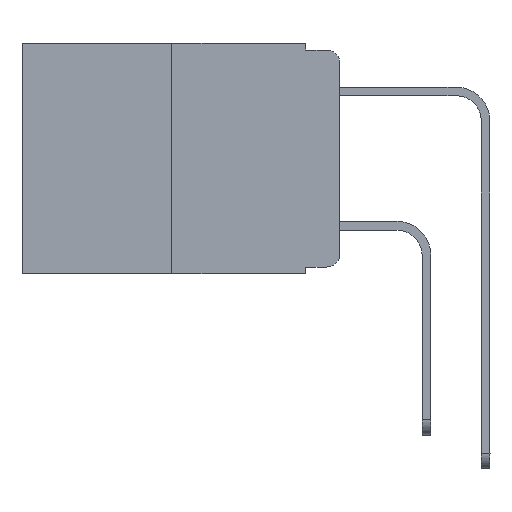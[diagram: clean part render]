
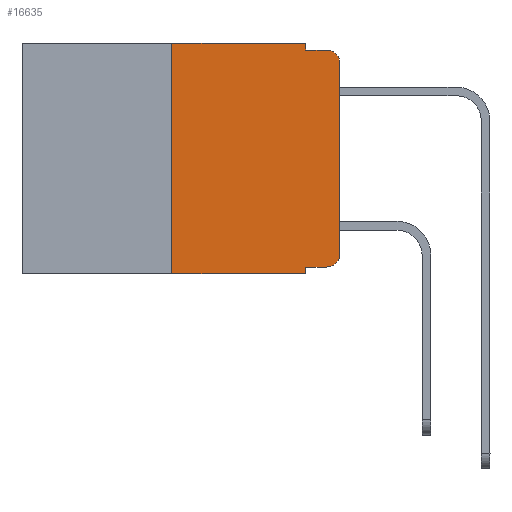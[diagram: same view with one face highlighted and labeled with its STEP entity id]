
A CAD part, left-side view. The second image highlights one B-rep face of the part: STEP entity #16635.
In plain terms, the highlighted planar face has unit normal (-1, 0, 0).
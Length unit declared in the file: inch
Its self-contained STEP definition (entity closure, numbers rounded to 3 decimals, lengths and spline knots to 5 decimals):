
#30 = ORIENTED_EDGE ( 'NONE', *, *, #8420, .T. ) ;
#124 = EDGE_CURVE ( 'NONE', #16669, #15917, #20163, .T. ) ;
#125 = DIRECTION ( 'NONE',  ( 0., 0., 1. ) ) ;
#176 = CARTESIAN_POINT ( 'NONE',  ( 0., 0.051, -0.01 ) ) ;
#660 = ORIENTED_EDGE ( 'NONE', *, *, #124, .T. ) ;
#1376 = CARTESIAN_POINT ( 'NONE',  ( 0., 0.25, 0. ) ) ;
#1667 = CARTESIAN_POINT ( 'NONE',  ( 0., 0.02, -0.313 ) ) ;
#3155 = CARTESIAN_POINT ( 'NONE',  ( 0., 0.051, 0. ) ) ;
#3241 = CARTESIAN_POINT ( 'NONE',  ( 0., 0.051, -0.343 ) ) ;
#3361 = LINE ( 'NONE', #5131, #3373 ) ;
#3373 = VECTOR ( 'NONE', #14288, 39.37008 ) ;
#3450 = DIRECTION ( 'NONE',  ( 1., 0., 0. ) ) ;
#3804 = VERTEX_POINT ( 'NONE', #176 ) ;
#4128 = DIRECTION ( 'NONE',  ( 0., -1., 0. ) ) ;
#4279 = EDGE_CURVE ( 'NONE', #8288, #5903, #12335, .T. ) ;
#4603 = VERTEX_POINT ( 'NONE', #13559 ) ;
#4614 = DIRECTION ( 'NONE',  ( 0., 0., -1. ) ) ;
#4744 = DIRECTION ( 'NONE',  ( 0., 0., -1. ) ) ;
#4758 = DIRECTION ( 'NONE',  ( 0., 0., 1. ) ) ;
#4771 = CARTESIAN_POINT ( 'NONE',  ( 0., 0.051, -0.333 ) ) ;
#5011 = PLANE ( 'NONE',  #13965 ) ;
#5131 = CARTESIAN_POINT ( 'NONE',  ( 0., 0.051, -0.01 ) ) ;
#5778 = AXIS2_PLACEMENT_3D ( 'NONE', #6007, #12176, #4744 ) ;
#5903 = VERTEX_POINT ( 'NONE', #3241 ) ;
#5946 = EDGE_CURVE ( 'NONE', #18652, #8633, #12513, .T. ) ;
#6007 = CARTESIAN_POINT ( 'NONE',  ( 0., 0.02, -0.03 ) ) ;
#6169 = EDGE_CURVE ( 'NONE', #15917, #17585, #12990, .T. ) ;
#6672 = EDGE_LOOP ( 'NONE', ( #660, #14178, #7880, #9277, #15893, #14570, #6991, #7124, #15206, #30 ) ) ;
#6991 = ORIENTED_EDGE ( 'NONE', *, *, #9196, .T. ) ;
#7124 = ORIENTED_EDGE ( 'NONE', *, *, #4279, .F. ) ;
#7330 = LINE ( 'NONE', #19630, #10176 ) ;
#7664 = CARTESIAN_POINT ( 'NONE',  ( 0., 0.25, -0.343 ) ) ;
#7880 = ORIENTED_EDGE ( 'NONE', *, *, #9917, .F. ) ;
#7937 = CARTESIAN_POINT ( 'NONE',  ( 0., 0.02, -0.01 ) ) ;
#8288 = VERTEX_POINT ( 'NONE', #16791 ) ;
#8420 = EDGE_CURVE ( 'NONE', #15781, #16669, #13388, .T. ) ;
#8600 = CARTESIAN_POINT ( 'NONE',  ( 0., 0., -0.313 ) ) ;
#8633 = VERTEX_POINT ( 'NONE', #11383 ) ;
#9075 = CARTESIAN_POINT ( 'NONE',  ( 0., 0.473, -0.343 ) ) ;
#9170 = EDGE_CURVE ( 'NONE', #8633, #4603, #7330, .T. ) ;
#9196 = EDGE_CURVE ( 'NONE', #18652, #5903, #16712, .T. ) ;
#9277 = ORIENTED_EDGE ( 'NONE', *, *, #15450, .F. ) ;
#9739 = DIRECTION ( 'NONE',  ( 0., 0., -1. ) ) ;
#9917 = EDGE_CURVE ( 'NONE', #3804, #17585, #3361, .T. ) ;
#10026 = VECTOR ( 'NONE', #11053, 39.37008 ) ;
#10176 = VECTOR ( 'NONE', #20034, 39.37008 ) ;
#10424 = AXIS2_PLACEMENT_3D ( 'NONE', #1667, #20210, #16883 ) ;
#11053 = DIRECTION ( 'NONE',  ( 0., -1., 0. ) ) ;
#11383 = CARTESIAN_POINT ( 'NONE',  ( 0., 0.25, 0. ) ) ;
#12176 = DIRECTION ( 'NONE',  ( -1., 0., 0. ) ) ;
#12335 = LINE ( 'NONE', #3155, #20222 ) ;
#12513 = LINE ( 'NONE', #1376, #14949 ) ;
#12990 = CIRCLE ( 'NONE', #5778, 0.02 ) ;
#13325 = CARTESIAN_POINT ( 'NONE',  ( 0., 0.051, 0. ) ) ;
#13388 = CIRCLE ( 'NONE', #10424, 0.02 ) ;
#13559 = CARTESIAN_POINT ( 'NONE',  ( 0., 0.051, 0. ) ) ;
#13585 = VECTOR ( 'NONE', #14992, 39.37008 ) ;
#13965 = AXIS2_PLACEMENT_3D ( 'NONE', #17584, #3450, #9739 ) ;
#14035 = CARTESIAN_POINT ( 'NONE',  ( 0., 0., 0. ) ) ;
#14117 = VECTOR ( 'NONE', #4128, 39.37008 ) ;
#14178 = ORIENTED_EDGE ( 'NONE', *, *, #6169, .T. ) ;
#14288 = DIRECTION ( 'NONE',  ( 0., -1., 0. ) ) ;
#14570 = ORIENTED_EDGE ( 'NONE', *, *, #5946, .F. ) ;
#14949 = VECTOR ( 'NONE', #125, 39.37008 ) ;
#14992 = DIRECTION ( 'NONE',  ( 0., 0., -1. ) ) ;
#15206 = ORIENTED_EDGE ( 'NONE', *, *, #17102, .T. ) ;
#15270 = CARTESIAN_POINT ( 'NONE',  ( 0., 0., -0.03 ) ) ;
#15450 = EDGE_CURVE ( 'NONE', #4603, #3804, #19770, .T. ) ;
#15781 = VERTEX_POINT ( 'NONE', #16013 ) ;
#15893 = ORIENTED_EDGE ( 'NONE', *, *, #9170, .F. ) ;
#15917 = VERTEX_POINT ( 'NONE', #15270 ) ;
#16013 = CARTESIAN_POINT ( 'NONE',  ( 0., 0.02, -0.333 ) ) ;
#16635 = ADVANCED_FACE ( 'NONE', ( #19147 ), #5011, .F. ) ;
#16669 = VERTEX_POINT ( 'NONE', #8600 ) ;
#16712 = LINE ( 'NONE', #9075, #14117 ) ;
#16791 = CARTESIAN_POINT ( 'NONE',  ( 0., 0.051, -0.333 ) ) ;
#16883 = DIRECTION ( 'NONE',  ( 0., 0., -1. ) ) ;
#17102 = EDGE_CURVE ( 'NONE', #8288, #15781, #18912, .T. ) ;
#17584 = CARTESIAN_POINT ( 'NONE',  ( 0., 0.473, 0. ) ) ;
#17585 = VERTEX_POINT ( 'NONE', #7937 ) ;
#17977 = VECTOR ( 'NONE', #4758, 39.37008 ) ;
#18652 = VERTEX_POINT ( 'NONE', #7664 ) ;
#18912 = LINE ( 'NONE', #4771, #10026 ) ;
#19147 = FACE_OUTER_BOUND ( 'NONE', #6672, .T. ) ;
#19630 = CARTESIAN_POINT ( 'NONE',  ( 0., 0.473, 0. ) ) ;
#19770 = LINE ( 'NONE', #13325, #13585 ) ;
#20034 = DIRECTION ( 'NONE',  ( 0., -1., 0. ) ) ;
#20163 = LINE ( 'NONE', #14035, #17977 ) ;
#20210 = DIRECTION ( 'NONE',  ( -1., 0., 0. ) ) ;
#20222 = VECTOR ( 'NONE', #4614, 39.37008 ) ;
